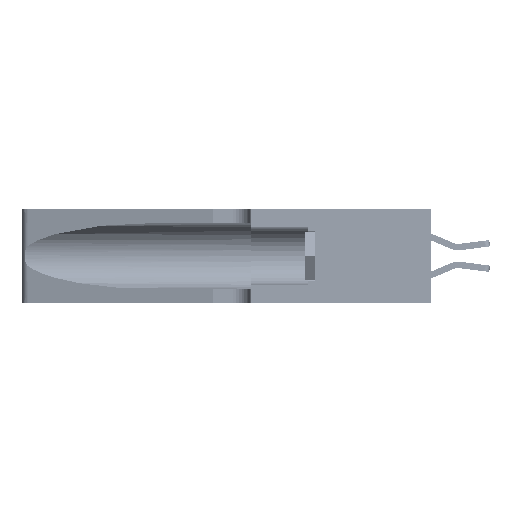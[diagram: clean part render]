
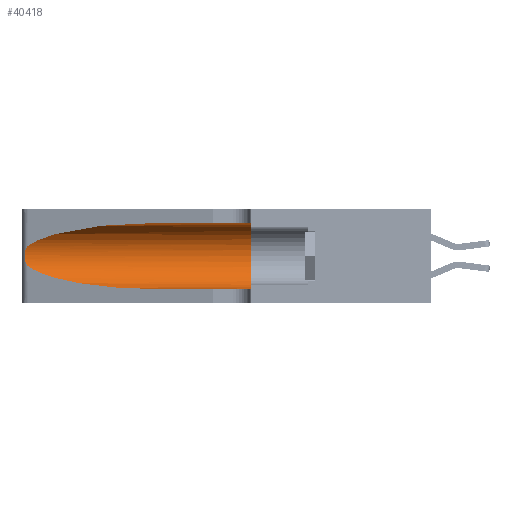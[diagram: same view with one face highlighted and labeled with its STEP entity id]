
A CAD part, left-side view. The second image highlights one B-rep face of the part: STEP entity #40418.
In plain terms, the highlighted cylindrical face has radius 3.308 mm (diameter 6.617 mm), a partial arc.
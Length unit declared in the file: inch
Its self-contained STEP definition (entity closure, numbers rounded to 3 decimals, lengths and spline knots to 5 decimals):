
#5 = DIRECTION ( 'NONE',  ( 0., -1., 0. ) ) ;
#2744 = CARTESIAN_POINT ( 'NONE',  ( 0.25487, 1.22718, 0.14631 ) ) ;
#2858 = EDGE_CURVE ( 'NONE', #25889, #19406, #17700, .T. ) ;
#2980 = VERTEX_POINT ( 'NONE', #8248 ) ;
#3131 = CARTESIAN_POINT ( 'NONE',  ( 0.25639, 1.23184, 0.21858 ) ) ;
#3780 = CARTESIAN_POINT ( 'NONE',  ( 0.25789, 1.23486, 0.15765 ) ) ;
#3820 = CARTESIAN_POINT ( 'NONE',  ( 0.1305, 0.35, 0.185 ) ) ;
#3965 = CARTESIAN_POINT ( 'NONE',  ( 0.25787, 1.23484, 0.2124 ) ) ;
#4687 = EDGE_CURVE ( 'NONE', #2980, #32016, #12459, .T. ) ;
#6231 = CARTESIAN_POINT ( 'NONE',  ( 0.25487, 1.22718, 0.22369 ) ) ;
#6289 = CARTESIAN_POINT ( 'NONE',  ( 0.1305, 0.72297, 0.05475 ) ) ;
#6646 = DIRECTION ( 'NONE',  ( 0., 0., -1. ) ) ;
#6953 = ORIENTED_EDGE ( 'NONE', *, *, #35137, .F. ) ;
#7192 = VERTEX_POINT ( 'NONE', #25508 ) ;
#8248 = CARTESIAN_POINT ( 'NONE',  ( 0.1305, 0.72297, 0.31525 ) ) ;
#8458 = ORIENTED_EDGE ( 'NONE', *, *, #36257, .T. ) ;
#8791 = CARTESIAN_POINT ( 'NONE',  ( 0.18966, 0.96281, 0.31525 ) ) ;
#10728 = FACE_OUTER_BOUND ( 'NONE', #37647, .T. ) ;
#11833 = CYLINDRICAL_SURFACE ( 'NONE', #15642, 0.13025 ) ;
#12459 = LINE ( 'NONE', #35914, #29511 ) ;
#13312 = EDGE_CURVE ( 'NONE', #31683, #7192, #34411, .T. ) ;
#13572 = EDGE_CURVE ( 'NONE', #2980, #25889, #36969, .T. ) ;
#13626 = CARTESIAN_POINT ( 'NONE',  ( 0.25487, 1.22718, 0.22369 ) ) ;
#13790 = VECTOR ( 'NONE', #20004, 39.37008 ) ;
#14994 = CARTESIAN_POINT ( 'NONE',  ( 0.26017, 1.23833, 0.17102 ) ) ;
#15609 = CARTESIAN_POINT ( 'NONE',  ( 0.2373, 1.15595, 0.28018 ) ) ;
#15642 = AXIS2_PLACEMENT_3D ( 'NONE', #26734, #5, #6646 ) ;
#17700 = B_SPLINE_CURVE_WITH_KNOTS ( 'NONE', 3,
 ( #13626, #26534, #3131, #3965, #33669, #27383, #37298, #37767, #14994, #25417, #3780, #42701, #36777, #21153 ),
 .UNSPECIFIED., .F., .F.,
 ( 4, 2, 2, 2, 2, 2, 4 ),
 ( 0., 0.00027, 0.00053, 0.00107, 0.0016, 0.00187, 0.00214 ),
 .UNSPECIFIED. ) ;
#19406 = VERTEX_POINT ( 'NONE', #25350 ) ;
#20004 = DIRECTION ( 'NONE',  ( 0., -1., 0. ) ) ;
#20613 = DIRECTION ( 'NONE',  ( 0., 0., 1. ) ) ;
#21153 = CARTESIAN_POINT ( 'NONE',  ( 0.25487, 1.22718, 0.14631 ) ) ;
#22720 = AXIS2_PLACEMENT_3D ( 'NONE', #3820, #33675, #20613 ) ;
#24685 = ORIENTED_EDGE ( 'NONE', *, *, #13312, .T. ) ;
#25350 = CARTESIAN_POINT ( 'NONE',  ( 0.25487, 1.22718, 0.14631 ) ) ;
#25417 = CARTESIAN_POINT ( 'NONE',  ( 0.25856, 1.23593, 0.16098 ) ) ;
#25508 = CARTESIAN_POINT ( 'NONE',  ( 0.1305, 0.35, 0.05475 ) ) ;
#25889 = VERTEX_POINT ( 'NONE', #6231 ) ;
#26534 = CARTESIAN_POINT ( 'NONE',  ( 0.25555, 1.22994, 0.2215 ) ) ;
#26734 = CARTESIAN_POINT ( 'NONE',  ( 0.1305, 1.61858, 0.185 ) ) ;
#27383 = CARTESIAN_POINT ( 'NONE',  ( 0.26018, 1.23835, 0.19895 ) ) ;
#28590 = CARTESIAN_POINT ( 'NONE',  ( 0.1305, 0.72297, 0.31525 ) ) ;
#28613 = ORIENTED_EDGE ( 'NONE', *, *, #13572, .T. ) ;
#29220 = CARTESIAN_POINT ( 'NONE',  ( 0.18966, 0.96281, 0.05475 ) ) ;
#29511 = VECTOR ( 'NONE', #36206, 39.37008 ) ;
#31626 = CIRCLE ( 'NONE', #22720, 0.13025 ) ;
#31683 = VERTEX_POINT ( 'NONE', #6289 ) ;
#32016 = VERTEX_POINT ( 'NONE', #37859 ) ;
#32376 = CARTESIAN_POINT ( 'NONE',  ( 0.1305, 1.61858, 0.05475 ) ) ;
#32482 = CARTESIAN_POINT ( 'NONE',  ( 0.1305, 0.72297, 0.05475 ) ) ;
#33669 = CARTESIAN_POINT ( 'NONE',  ( 0.25854, 1.2359, 0.20912 ) ) ;
#33675 = DIRECTION ( 'NONE',  ( 0., 1., 0. ) ) ;
#34411 = LINE ( 'NONE', #32376, #13790 ) ;
#35137 = EDGE_CURVE ( 'NONE', #32016, #7192, #31626, .T. ) ;
#35584 = CARTESIAN_POINT ( 'NONE',  ( 0.25487, 1.22718, 0.22369 ) ) ;
#35914 = CARTESIAN_POINT ( 'NONE',  ( 0.1305, 1.61858, 0.31525 ) ) ;
#36206 = DIRECTION ( 'NONE',  ( 0., -1., 0. ) ) ;
#36257 = EDGE_CURVE ( 'NONE', #19406, #31683, #38894, .T. ) ;
#36777 = CARTESIAN_POINT ( 'NONE',  ( 0.25555, 1.22993, 0.14849 ) ) ;
#36969 =( BOUNDED_CURVE ( )  B_SPLINE_CURVE ( 3, ( #28590, #8791, #15609, #35584 ),
 .UNSPECIFIED., .F., .T. ) 
 B_SPLINE_CURVE_WITH_KNOTS ( ( 4, 4 ),
 ( 1.5708, 2.84003 ),
 .UNSPECIFIED. ) 
 CURVE ( )  GEOMETRIC_REPRESENTATION_ITEM ( )  RATIONAL_B_SPLINE_CURVE ( ( 1., 0.87, 0.87, 1. ) ) 
 REPRESENTATION_ITEM ( '' )  );
#37298 = CARTESIAN_POINT ( 'NONE',  ( 0.26075, 1.23896, 0.19203 ) ) ;
#37647 = EDGE_LOOP ( 'NONE', ( #28613, #39675, #8458, #24685, #6953, #40924 ) ) ;
#37767 = CARTESIAN_POINT ( 'NONE',  ( 0.26075, 1.23896, 0.178 ) ) ;
#37859 = CARTESIAN_POINT ( 'NONE',  ( 0.1305, 0.35, 0.31525 ) ) ;
#38894 =( BOUNDED_CURVE ( )  B_SPLINE_CURVE ( 3, ( #2744, #39459, #29220, #32482 ),
 .UNSPECIFIED., .F., .F. ) 
 B_SPLINE_CURVE_WITH_KNOTS ( ( 4, 4 ),
 ( 3.44316, 4.71239 ),
 .UNSPECIFIED. ) 
 CURVE ( )  GEOMETRIC_REPRESENTATION_ITEM ( )  RATIONAL_B_SPLINE_CURVE ( ( 1., 0.87, 0.87, 1. ) ) 
 REPRESENTATION_ITEM ( '' )  );
#39459 = CARTESIAN_POINT ( 'NONE',  ( 0.2373, 1.15595, 0.08982 ) ) ;
#39675 = ORIENTED_EDGE ( 'NONE', *, *, #2858, .T. ) ;
#40418 = ADVANCED_FACE ( 'NONE', ( #10728 ), #11833, .F. ) ;
#40924 = ORIENTED_EDGE ( 'NONE', *, *, #4687, .F. ) ;
#42701 = CARTESIAN_POINT ( 'NONE',  ( 0.25639, 1.23186, 0.15144 ) ) ;
